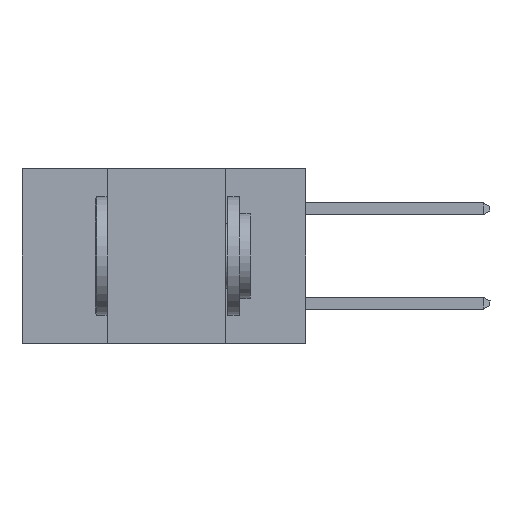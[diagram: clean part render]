
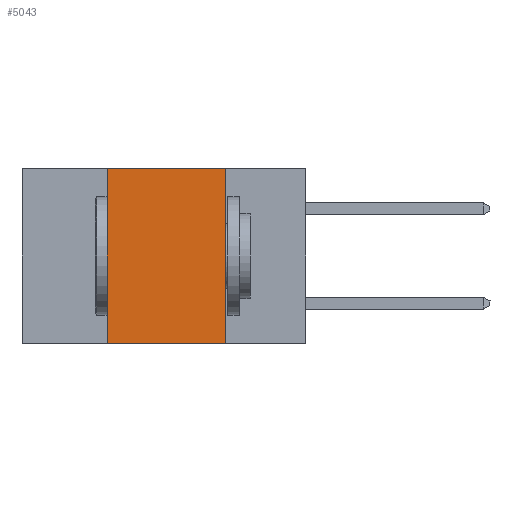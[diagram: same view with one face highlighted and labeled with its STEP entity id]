
A CAD part, left-side view. The second image highlights one B-rep face of the part: STEP entity #5043.
In plain terms, the highlighted planar face has unit normal (-1, 0, 0).
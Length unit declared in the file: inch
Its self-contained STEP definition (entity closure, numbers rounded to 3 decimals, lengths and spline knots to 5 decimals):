
#31 = CARTESIAN_POINT ( 'NONE',  ( 0., 0.6, 0. ) ) ;
#66 = VECTOR ( 'NONE', #10686, 39.37008 ) ;
#449 = CARTESIAN_POINT ( 'NONE',  ( 0., 0.17, 0. ) ) ;
#652 = ORIENTED_EDGE ( 'NONE', *, *, #12369, .T. ) ;
#1284 = VERTEX_POINT ( 'NONE', #12014 ) ;
#1636 = EDGE_CURVE ( 'NONE', #7811, #7835, #10248, .T. ) ;
#2130 = CARTESIAN_POINT ( 'NONE',  ( 0., 0.42, -0.37 ) ) ;
#2606 = ORIENTED_EDGE ( 'NONE', *, *, #1636, .F. ) ;
#2881 = EDGE_CURVE ( 'NONE', #1284, #7811, #8498, .T. ) ;
#3366 = DIRECTION ( 'NONE',  ( 0., 0., -1. ) ) ;
#3686 = DIRECTION ( 'NONE',  ( 0., 0., -1. ) ) ;
#3730 = VECTOR ( 'NONE', #6835, 39.37008 ) ;
#3810 = VECTOR ( 'NONE', #12329, 39.37008 ) ;
#4288 = CARTESIAN_POINT ( 'NONE',  ( 0., 0.17, 0. ) ) ;
#4717 = ORIENTED_EDGE ( 'NONE', *, *, #2881, .F. ) ;
#5043 = ADVANCED_FACE ( 'NONE', ( #7820 ), #11592, .F. ) ;
#5736 = CARTESIAN_POINT ( 'NONE',  ( 0., 0.6, 0. ) ) ;
#5752 = EDGE_CURVE ( 'NONE', #10359, #1284, #6441, .T. ) ;
#6441 = LINE ( 'NONE', #9401, #3810 ) ;
#6835 = DIRECTION ( 'NONE',  ( 0., -1., 0. ) ) ;
#7174 = CARTESIAN_POINT ( 'NONE',  ( 0., 0.17, -0.37 ) ) ;
#7811 = VERTEX_POINT ( 'NONE', #4288 ) ;
#7820 = FACE_OUTER_BOUND ( 'NONE', #8469, .T. ) ;
#7835 = VERTEX_POINT ( 'NONE', #7174 ) ;
#8469 = EDGE_LOOP ( 'NONE', ( #2606, #4717, #8578, #652 ) ) ;
#8498 = LINE ( 'NONE', #31, #66 ) ;
#8578 = ORIENTED_EDGE ( 'NONE', *, *, #5752, .F. ) ;
#9264 = AXIS2_PLACEMENT_3D ( 'NONE', #5736, #9596, #3686 ) ;
#9401 = CARTESIAN_POINT ( 'NONE',  ( 0., 0.42, 0. ) ) ;
#9596 = DIRECTION ( 'NONE',  ( 1., 0., 0. ) ) ;
#10248 = LINE ( 'NONE', #449, #11921 ) ;
#10359 = VERTEX_POINT ( 'NONE', #2130 ) ;
#10363 = LINE ( 'NONE', #10776, #3730 ) ;
#10686 = DIRECTION ( 'NONE',  ( 0., -1., 0. ) ) ;
#10776 = CARTESIAN_POINT ( 'NONE',  ( 0., 0.6, -0.37 ) ) ;
#11592 = PLANE ( 'NONE',  #9264 ) ;
#11921 = VECTOR ( 'NONE', #3366, 39.37008 ) ;
#12014 = CARTESIAN_POINT ( 'NONE',  ( 0., 0.42, 0. ) ) ;
#12329 = DIRECTION ( 'NONE',  ( 0., 0., 1. ) ) ;
#12369 = EDGE_CURVE ( 'NONE', #10359, #7835, #10363, .T. ) ;
